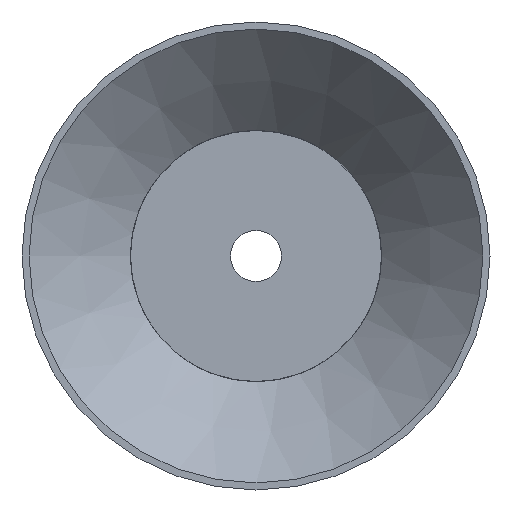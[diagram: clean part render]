
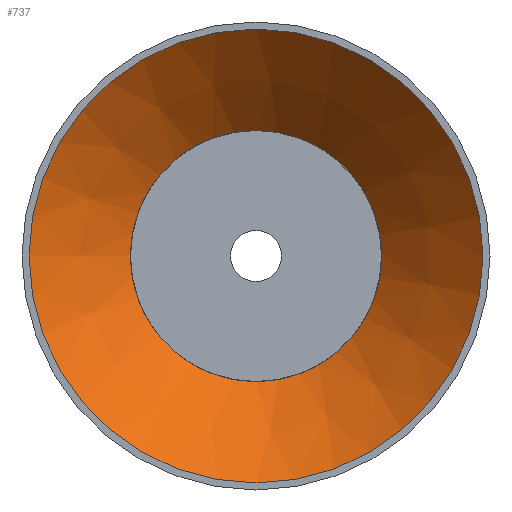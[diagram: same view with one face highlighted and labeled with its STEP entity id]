
A CAD part, front view. The second image highlights one B-rep face of the part: STEP entity #737.
In plain terms, the highlighted conical face has half-angle 44.602 degrees and reference radius 31.559 mm.
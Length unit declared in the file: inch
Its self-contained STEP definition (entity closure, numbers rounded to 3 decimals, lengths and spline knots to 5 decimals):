
#127=FACE_OUTER_BOUND('',#163,.T.);
#163=EDGE_LOOP('',(#489,#490,#491,#492,#493,#494));
#206=LINE('',#976,#228);
#228=VECTOR('',#846,1.2425);
#250=CIRCLE('',#788,1.6);
#251=CIRCLE('',#789,0.885);
#252=CIRCLE('',#790,0.885);
#253=CIRCLE('',#791,1.6);
#280=VERTEX_POINT('',#972);
#281=VERTEX_POINT('',#973);
#282=VERTEX_POINT('',#975);
#283=VERTEX_POINT('',#977);
#366=EDGE_CURVE('',#280,#281,#250,.T.);
#367=EDGE_CURVE('',#281,#282,#206,.T.);
#368=EDGE_CURVE('',#283,#282,#251,.T.);
#369=EDGE_CURVE('',#282,#283,#252,.T.);
#370=EDGE_CURVE('',#281,#280,#253,.T.);
#489=ORIENTED_EDGE('',*,*,#366,.T.);
#490=ORIENTED_EDGE('',*,*,#367,.T.);
#491=ORIENTED_EDGE('',*,*,#368,.F.);
#492=ORIENTED_EDGE('',*,*,#369,.F.);
#493=ORIENTED_EDGE('',*,*,#367,.F.);
#494=ORIENTED_EDGE('',*,*,#370,.T.);
#735=CONICAL_SURFACE('',#787,1.2425,0.778);
#737=ADVANCED_FACE('',(#127),#735,.F.);
#787=AXIS2_PLACEMENT_3D('',#971,#842,#843);
#788=AXIS2_PLACEMENT_3D('',#974,#844,#845);
#789=AXIS2_PLACEMENT_3D('',#978,#847,#848);
#790=AXIS2_PLACEMENT_3D('',#979,#849,#850);
#791=AXIS2_PLACEMENT_3D('',#980,#851,#852);
#842=DIRECTION('center_axis',(0.,-1.,0.));
#843=DIRECTION('ref_axis',(1.,0.,0.));
#844=DIRECTION('center_axis',(0.,-1.,0.));
#845=DIRECTION('ref_axis',(1.,0.,0.));
#846=DIRECTION('',(0.702,0.712,0.));
#847=DIRECTION('center_axis',(0.,-1.,0.));
#848=DIRECTION('ref_axis',(1.,0.,0.));
#849=DIRECTION('center_axis',(0.,-1.,0.));
#850=DIRECTION('ref_axis',(1.,0.,0.));
#851=DIRECTION('center_axis',(0.,-1.,0.));
#852=DIRECTION('ref_axis',(1.,0.,0.));
#971=CARTESIAN_POINT('Origin',(0.,0.3625,0.));
#972=CARTESIAN_POINT('',(1.6,0.,0.));
#973=CARTESIAN_POINT('',(-1.6,0.,0.));
#974=CARTESIAN_POINT('Origin',(0.,0.,0.));
#975=CARTESIAN_POINT('',(-0.885,0.725,0.));
#976=CARTESIAN_POINT('',(-1.2425,0.3625,0.));
#977=CARTESIAN_POINT('',(0.885,0.725,0.));
#978=CARTESIAN_POINT('Origin',(0.,0.725,0.));
#979=CARTESIAN_POINT('Origin',(0.,0.725,0.));
#980=CARTESIAN_POINT('Origin',(0.,0.,0.));
